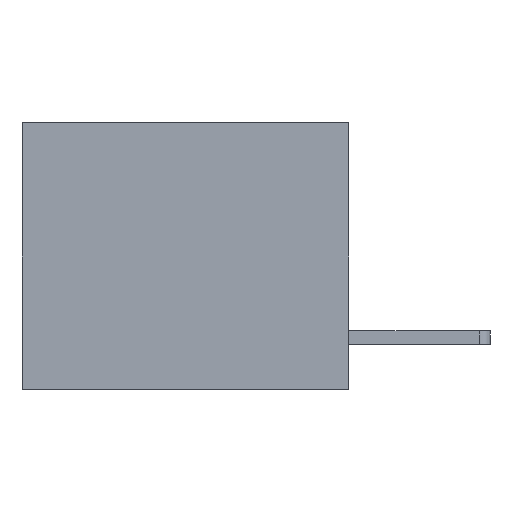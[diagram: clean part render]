
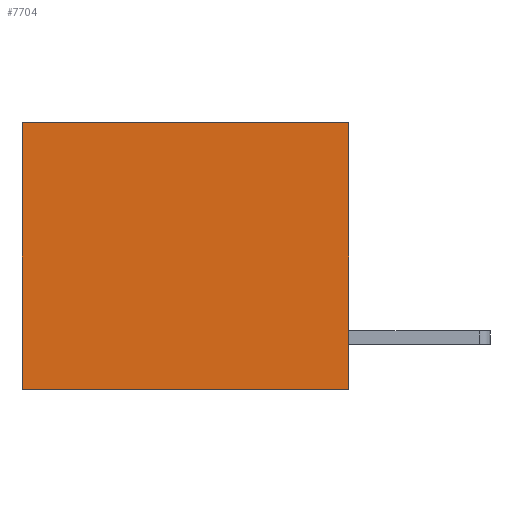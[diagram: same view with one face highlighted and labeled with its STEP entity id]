
A CAD part, left-side view. The second image highlights one B-rep face of the part: STEP entity #7704.
In plain terms, the highlighted planar face has unit normal (-1, 0, 0).
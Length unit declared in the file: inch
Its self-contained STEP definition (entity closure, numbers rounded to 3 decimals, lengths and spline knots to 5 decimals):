
#101 = LINE ( 'NONE', #3794, #4044 ) ;
#732 = DIRECTION ( 'NONE',  ( 0., 0., -1. ) ) ;
#960 = CARTESIAN_POINT ( 'NONE',  ( 0.3165, 0.6, -0.49 ) ) ;
#989 = CARTESIAN_POINT ( 'NONE',  ( 0.3165, 0.6, 0. ) ) ;
#1190 = PLANE ( 'NONE',  #2507 ) ;
#1268 = VERTEX_POINT ( 'NONE', #3846 ) ;
#1371 = CARTESIAN_POINT ( 'NONE',  ( 0.3165, 0., -0.49 ) ) ;
#2061 = CARTESIAN_POINT ( 'NONE',  ( 0.3165, 0., -0.49 ) ) ;
#2378 = FACE_OUTER_BOUND ( 'NONE', #8460, .T. ) ;
#2507 = AXIS2_PLACEMENT_3D ( 'NONE', #2650, #3412, #4992 ) ;
#2650 = CARTESIAN_POINT ( 'NONE',  ( 0.3165, 0., -0.49 ) ) ;
#3097 = CARTESIAN_POINT ( 'NONE',  ( 0.3165, 0., 0. ) ) ;
#3243 = EDGE_CURVE ( 'NONE', #1268, #6559, #6786, .T. ) ;
#3412 = DIRECTION ( 'NONE',  ( 1., 0., 0. ) ) ;
#3552 = LINE ( 'NONE', #1371, #7417 ) ;
#3794 = CARTESIAN_POINT ( 'NONE',  ( 0.3165, 0., 0. ) ) ;
#3832 = ORIENTED_EDGE ( 'NONE', *, *, #4905, .T. ) ;
#3846 = CARTESIAN_POINT ( 'NONE',  ( 0.3165, 0., -0.49 ) ) ;
#4044 = VECTOR ( 'NONE', #5292, 39.37008 ) ;
#4079 = VERTEX_POINT ( 'NONE', #989 ) ;
#4905 = EDGE_CURVE ( 'NONE', #4079, #6559, #9832, .T. ) ;
#4992 = DIRECTION ( 'NONE',  ( 0., 0., -1. ) ) ;
#5292 = DIRECTION ( 'NONE',  ( 0., 1., 0. ) ) ;
#5324 = ORIENTED_EDGE ( 'NONE', *, *, #9780, .F. ) ;
#6117 = CARTESIAN_POINT ( 'NONE',  ( 0.3165, 0.6, -0.49 ) ) ;
#6302 = VECTOR ( 'NONE', #7470, 39.37008 ) ;
#6334 = EDGE_CURVE ( 'NONE', #8573, #4079, #101, .T. ) ;
#6500 = VECTOR ( 'NONE', #9258, 39.37008 ) ;
#6559 = VERTEX_POINT ( 'NONE', #960 ) ;
#6786 = LINE ( 'NONE', #2061, #6302 ) ;
#6924 = ORIENTED_EDGE ( 'NONE', *, *, #6334, .T. ) ;
#7417 = VECTOR ( 'NONE', #732, 39.37008 ) ;
#7470 = DIRECTION ( 'NONE',  ( 0., 1., 0. ) ) ;
#7704 = ADVANCED_FACE ( 'NONE', ( #2378 ), #1190, .F. ) ;
#8460 = EDGE_LOOP ( 'NONE', ( #3832, #9213, #5324, #6924 ) ) ;
#8573 = VERTEX_POINT ( 'NONE', #3097 ) ;
#9213 = ORIENTED_EDGE ( 'NONE', *, *, #3243, .F. ) ;
#9258 = DIRECTION ( 'NONE',  ( 0., 0., -1. ) ) ;
#9780 = EDGE_CURVE ( 'NONE', #8573, #1268, #3552, .T. ) ;
#9832 = LINE ( 'NONE', #6117, #6500 ) ;
